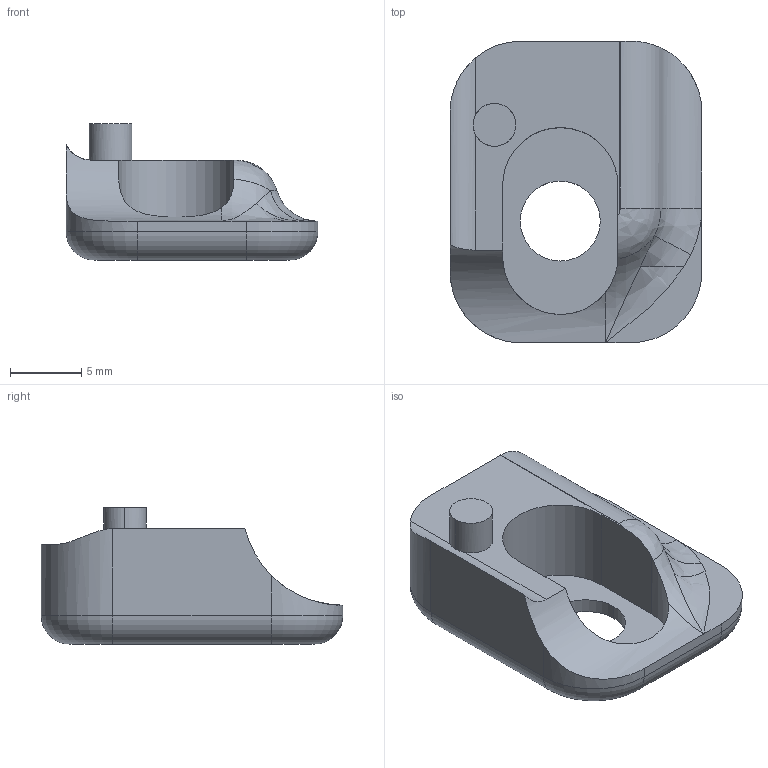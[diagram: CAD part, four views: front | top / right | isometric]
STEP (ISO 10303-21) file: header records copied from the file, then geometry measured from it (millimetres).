
FILE_DESCRIPTION (( 'STEP AP214' ), '1' );
FILE_NAME ('Hermes_Release_Cover.STEP', '2013-12-17T06:22:04', ( 'elpi' ), ( '' ), 'SwSTEP 2.0', 'SolidWorks 2013', '' );
FILE_SCHEMA (( 'AUTOMOTIVE_DESIGN' ));
Length unit declared in the file: millimetre
Products named in the file (1): Hermes_Release_Cover
Bounding box: 17.64 x 21.12 x 9.54 mm (x, y, z)
Volume: 1413.8 mm3; surface area: 1173.7 mm2
Topology: 1 solids, 1 shells, 39 faces, 99 edges, 61 vertices
Faces by surface type: cylinder 19, plane 11, torus 5, bspline 4
Entity records: 1587 total; most frequent: CARTESIAN_POINT 642, ORIENTED_EDGE 196, DIRECTION 186, EDGE_CURVE 98, AXIS2_PLACEMENT_3D 73, VERTEX_POINT 61, EDGE_LOOP 41, LINE 40
